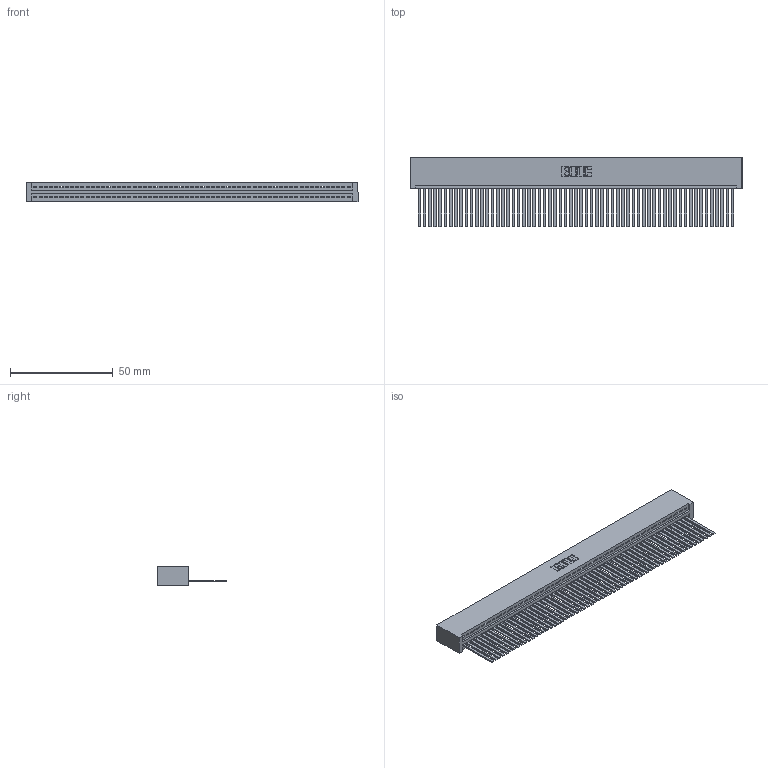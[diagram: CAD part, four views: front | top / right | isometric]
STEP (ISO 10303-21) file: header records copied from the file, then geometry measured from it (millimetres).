
FILE_DESCRIPTION (( 'STEP AP203' ), '1' );
FILE_NAME ('395-061-544-101.STEP', '2019-10-24T15:56:24', ( '' ), ( '' ), 'SwSTEP 2.0', 'SolidWorks 2016', '' );
FILE_SCHEMA (( 'CONFIG_CONTROL_DESIGN' ));
Length unit declared in the file: inch
Products named in the file (3): 345-292-001_345-293-144; 345 Part_No Mounting Lugs; 395-061-544-101
Assembly tree (62 placements, depth 2):
  395-061-544-101
    345 Part_No Mounting Lugs
    345-292-001_345-293-144  x61
Bounding box: 161.54 x 33.96 x 9.4 mm (x, y, z)
Volume: 16790.1 mm3; surface area: 24881.7 mm2
Topology: 62 solids, 62 shells, 3290 faces, 9955 edges, 6554 vertices
Faces by surface type: plane 2272, cylinder 1018
Entity records: 42891 total; most frequent: CARTESIAN_POINT 7435, ORIENTED_EDGE 7430, DIRECTION 6457, EDGE_CURVE 3715, LINE 3351, VECTOR 3351, VERTEX_POINT 2474, AXIS2_PLACEMENT_3D 1553
